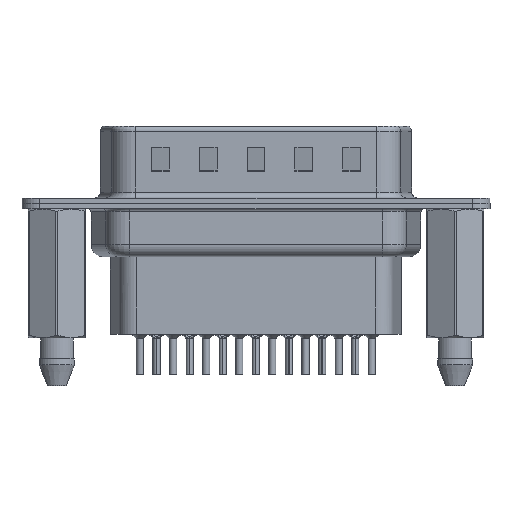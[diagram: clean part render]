
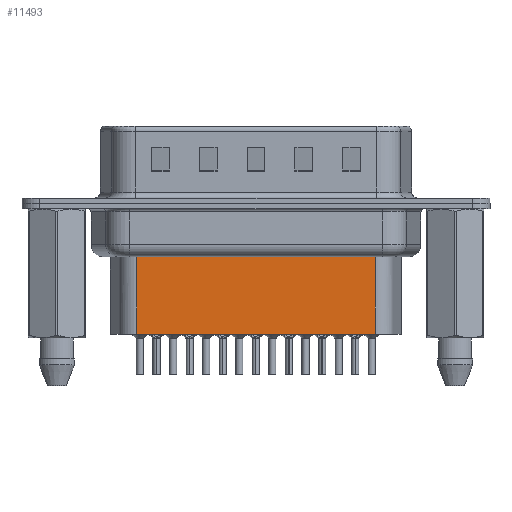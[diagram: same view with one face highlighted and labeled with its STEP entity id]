
A CAD part, front view. The second image highlights one B-rep face of the part: STEP entity #11493.
In plain terms, the highlighted planar face has unit normal (0, -1, 0).
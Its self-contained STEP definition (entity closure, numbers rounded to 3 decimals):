
#108 = VERTEX_POINT ( 'NONE', #21535 ) ;
#468 = LINE ( 'NONE', #10334, #8261 ) ;
#1439 = ORIENTED_EDGE ( 'NONE', *, *, #2492, .T. ) ;
#1535 = LINE ( 'NONE', #20417, #14982 ) ;
#2492 = EDGE_CURVE ( 'NONE', #18131, #11239, #1535, .T. ) ;
#3984 = CARTESIAN_POINT ( 'NONE',  ( 26.619, -3.5, -10.95 ) ) ;
#4123 = EDGE_CURVE ( 'NONE', #108, #18052, #13737, .T. ) ;
#4740 = LINE ( 'NONE', #12485, #20087 ) ;
#4853 = CARTESIAN_POINT ( 'NONE',  ( 6.681, -3.5, -10.95 ) ) ;
#6612 = VECTOR ( 'NONE', #17403, 1000. ) ;
#6664 = ORIENTED_EDGE ( 'NONE', *, *, #7297, .F. ) ;
#7297 = EDGE_CURVE ( 'NONE', #18052, #11239, #4740, .T. ) ;
#8261 = VECTOR ( 'NONE', #12117, 1000. ) ;
#8392 = CARTESIAN_POINT ( 'NONE',  ( 6.681, -3.5, -4.097 ) ) ;
#8760 = DIRECTION ( 'NONE',  ( 0., 0., -1. ) ) ;
#9779 = CARTESIAN_POINT ( 'NONE',  ( 26.619, -3.5, -3.1 ) ) ;
#10334 = CARTESIAN_POINT ( 'NONE',  ( 6.434, -3.5, -4.097 ) ) ;
#11239 = VERTEX_POINT ( 'NONE', #4853 ) ;
#11493 = ADVANCED_FACE ( 'NONE', ( #19681 ), #17918, .T. ) ;
#11944 = EDGE_LOOP ( 'NONE', ( #16545, #15135, #1439, #6664 ) ) ;
#12117 = DIRECTION ( 'NONE',  ( -1., 0., 0. ) ) ;
#12485 = CARTESIAN_POINT ( 'NONE',  ( 6.681, -3.5, -10.95 ) ) ;
#13737 = LINE ( 'NONE', #9779, #6612 ) ;
#14241 = DIRECTION ( 'NONE',  ( 1., 0., 0. ) ) ;
#14982 = VECTOR ( 'NONE', #8760, 1000. ) ;
#15135 = ORIENTED_EDGE ( 'NONE', *, *, #17776, .T. ) ;
#16157 = AXIS2_PLACEMENT_3D ( 'NONE', #21698, #20167, #14241 ) ;
#16545 = ORIENTED_EDGE ( 'NONE', *, *, #4123, .F. ) ;
#17403 = DIRECTION ( 'NONE',  ( 0., 0., -1. ) ) ;
#17776 = EDGE_CURVE ( 'NONE', #108, #18131, #468, .T. ) ;
#17918 = PLANE ( 'NONE',  #16157 ) ;
#18052 = VERTEX_POINT ( 'NONE', #3984 ) ;
#18131 = VERTEX_POINT ( 'NONE', #8392 ) ;
#19681 = FACE_OUTER_BOUND ( 'NONE', #11944, .T. ) ;
#20087 = VECTOR ( 'NONE', #24490, 1000. ) ;
#20167 = DIRECTION ( 'NONE',  ( 0., -1., 0. ) ) ;
#20417 = CARTESIAN_POINT ( 'NONE',  ( 6.681, -3.5, -3.1 ) ) ;
#21535 = CARTESIAN_POINT ( 'NONE',  ( 26.619, -3.5, -4.097 ) ) ;
#21698 = CARTESIAN_POINT ( 'NONE',  ( 6.681, -3.5, -3.1 ) ) ;
#24490 = DIRECTION ( 'NONE',  ( -1., 0., 0. ) ) ;
